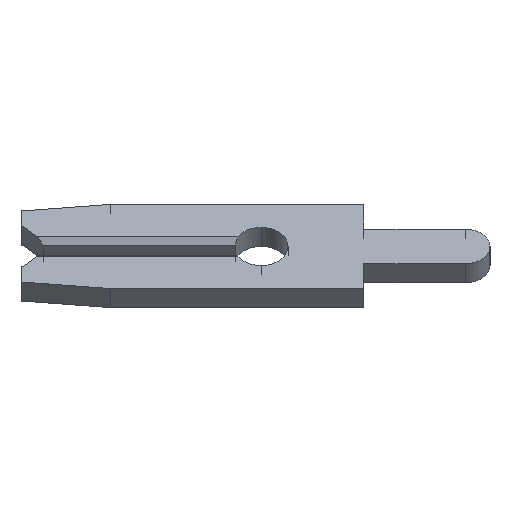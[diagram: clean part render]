
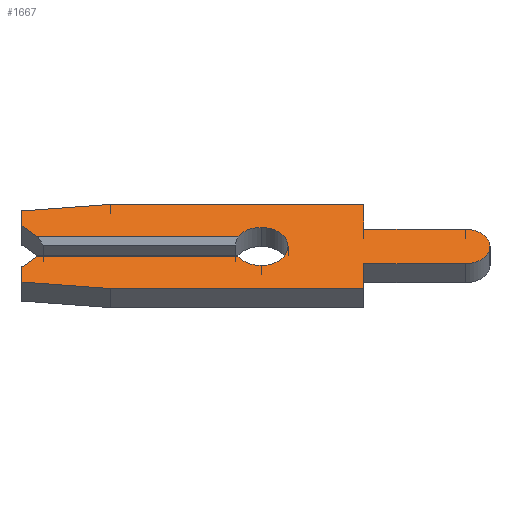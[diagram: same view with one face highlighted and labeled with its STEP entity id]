
A CAD part, left-side view. The second image highlights one B-rep face of the part: STEP entity #1667.
In plain terms, the highlighted face is planar.
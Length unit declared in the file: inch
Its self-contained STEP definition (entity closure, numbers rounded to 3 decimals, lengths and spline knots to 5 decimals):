
#4 = EDGE_CURVE ( 'NONE', #244, #461, #1239, .T. ) ;
#5 = VERTEX_POINT ( 'NONE', #1364 ) ;
#34 = CARTESIAN_POINT ( 'NONE',  ( -0.013, -0.099, -0.0235 ) ) ;
#36 = CARTESIAN_POINT ( 'NONE',  ( -0.013, 0.146, -0.0575 ) ) ;
#54 = VERTEX_POINT ( 'NONE', #1361 ) ;
#83 = EDGE_CURVE ( 'NONE', #1002, #1341, #1536, .T. ) ;
#96 = ORIENTED_EDGE ( 'NONE', *, *, #337, .F. ) ;
#134 = CARTESIAN_POINT ( 'NONE',  ( -0.013, 0.231, 0.028 ) ) ;
#136 = ORIENTED_EDGE ( 'NONE', *, *, #1131, .F. ) ;
#138 = CARTESIAN_POINT ( 'NONE',  ( -0.013, 0.231, 0.04857 ) ) ;
#140 = ORIENTED_EDGE ( 'NONE', *, *, #744, .F. ) ;
#153 = CARTESIAN_POINT ( 'NONE',  ( -0.013, 0., 0. ) ) ;
#181 = EDGE_CURVE ( 'NONE', #1184, #1570, #1102, .T. ) ;
#193 = VERTEX_POINT ( 'NONE', #850 ) ;
#195 = LINE ( 'NONE', #522, #796 ) ;
#197 = DIRECTION ( 'NONE',  ( 0., 0., -1. ) ) ;
#204 = CARTESIAN_POINT ( 'NONE',  ( -0.013, -0.1975, -0.0235 ) ) ;
#235 = ORIENTED_EDGE ( 'NONE', *, *, #1245, .F. ) ;
#244 = VERTEX_POINT ( 'NONE', #204 ) ;
#266 = CARTESIAN_POINT ( 'NONE',  ( -0.013, 0., 0. ) ) ;
#281 = EDGE_CURVE ( 'NONE', #320, #244, #333, .T. ) ;
#283 = ORIENTED_EDGE ( 'NONE', *, *, #181, .F. ) ;
#285 = ORIENTED_EDGE ( 'NONE', *, *, #4, .F. ) ;
#316 = VECTOR ( 'NONE', #1560, 39.37008 ) ;
#320 = VERTEX_POINT ( 'NONE', #1524 ) ;
#322 = LINE ( 'NONE', #1227, #638 ) ;
#330 = EDGE_CURVE ( 'NONE', #461, #592, #766, .T. ) ;
#333 = CIRCLE ( 'NONE', #1401, 0.0235 ) ;
#337 = EDGE_CURVE ( 'NONE', #659, #320, #1081, .T. ) ;
#347 = DIRECTION ( 'NONE',  ( 1., 0., 0. ) ) ;
#358 = LINE ( 'NONE', #507, #316 ) ;
#382 = VECTOR ( 'NONE', #597, 39.37008 ) ;
#411 = VECTOR ( 'NONE', #786, 39.37008 ) ;
#420 = VERTEX_POINT ( 'NONE', #1701 ) ;
#424 = EDGE_CURVE ( 'NONE', #1570, #1647, #358, .T. ) ;
#461 = VERTEX_POINT ( 'NONE', #1427 ) ;
#467 = CARTESIAN_POINT ( 'NONE',  ( -0.013, 0.231, -0.04857 ) ) ;
#479 = DIRECTION ( 'NONE',  ( 1., 0., 0. ) ) ;
#488 = ORIENTED_EDGE ( 'NONE', *, *, #330, .F. ) ;
#490 = LINE ( 'NONE', #134, #1108 ) ;
#505 = CARTESIAN_POINT ( 'NONE',  ( -0.013, 0.216, -0.013 ) ) ;
#507 = CARTESIAN_POINT ( 'NONE',  ( -0.013, 0.231, -0.028 ) ) ;
#515 = LINE ( 'NONE', #138, #574 ) ;
#522 = CARTESIAN_POINT ( 'NONE',  ( -0.013, 0.146, 0.0575 ) ) ;
#531 = DIRECTION ( 'NONE',  ( -1., 0., 0. ) ) ;
#536 = DIRECTION ( 'NONE',  ( 0., 0., -1. ) ) ;
#545 = AXIS2_PLACEMENT_3D ( 'NONE', #936, #1602, #536 ) ;
#570 = CARTESIAN_POINT ( 'NONE',  ( -0.013, 0.231, 0.013 ) ) ;
#574 = VECTOR ( 'NONE', #1463, 39.37008 ) ;
#585 = ORIENTED_EDGE ( 'NONE', *, *, #839, .F. ) ;
#591 = ORIENTED_EDGE ( 'NONE', *, *, #1204, .F. ) ;
#592 = VERTEX_POINT ( 'NONE', #619 ) ;
#597 = DIRECTION ( 'NONE',  ( 0., 0.995, 0.105 ) ) ;
#602 = CARTESIAN_POINT ( 'NONE',  ( -0.013, -0.099, 0.0235 ) ) ;
#619 = CARTESIAN_POINT ( 'NONE',  ( -0.013, -0.099, -0.0575 ) ) ;
#622 = ORIENTED_EDGE ( 'NONE', *, *, #424, .F. ) ;
#638 = VECTOR ( 'NONE', #967, 39.37008 ) ;
#659 = VERTEX_POINT ( 'NONE', #1454 ) ;
#671 = EDGE_CURVE ( 'NONE', #1002, #193, #1617, .T. ) ;
#677 = DIRECTION ( 'NONE',  ( 0., 0., -1. ) ) ;
#680 = ORIENTED_EDGE ( 'NONE', *, *, #1024, .F. ) ;
#689 = CARTESIAN_POINT ( 'NONE',  ( -0.013, 0., -0.026 ) ) ;
#701 = DIRECTION ( 'NONE',  ( 0., -1., 0. ) ) ;
#708 = ORIENTED_EDGE ( 'NONE', *, *, #1312, .F. ) ;
#711 = CIRCLE ( 'NONE', #1095, 0.026 ) ;
#744 = EDGE_CURVE ( 'NONE', #420, #5, #195, .T. ) ;
#766 = LINE ( 'NONE', #1660, #1497 ) ;
#786 = DIRECTION ( 'NONE',  ( 0., 0.707, 0.707 ) ) ;
#794 = CARTESIAN_POINT ( 'NONE',  ( -0.013, 0.231, 0.04857 ) ) ;
#796 = VECTOR ( 'NONE', #823, 39.37008 ) ;
#801 = DIRECTION ( 'NONE',  ( 0., -1., 0. ) ) ;
#819 = DIRECTION ( 'NONE',  ( -1., 0., 0. ) ) ;
#823 = DIRECTION ( 'NONE',  ( 0., -1., 0. ) ) ;
#837 = FACE_OUTER_BOUND ( 'NONE', #1158, .T. ) ;
#839 = EDGE_CURVE ( 'NONE', #5, #659, #902, .T. ) ;
#850 = CARTESIAN_POINT ( 'NONE',  ( -0.013, 0.231, 0.028 ) ) ;
#854 = ORIENTED_EDGE ( 'NONE', *, *, #892, .F. ) ;
#858 = DIRECTION ( 'NONE',  ( 0., 0., -1. ) ) ;
#867 = CARTESIAN_POINT ( 'NONE',  ( -0.013, -0.1975, 0. ) ) ;
#874 = DIRECTION ( 'NONE',  ( 0., -1., 0. ) ) ;
#888 = VECTOR ( 'NONE', #1644, 39.37008 ) ;
#892 = EDGE_CURVE ( 'NONE', #1647, #897, #1071, .T. ) ;
#897 = VERTEX_POINT ( 'NONE', #505 ) ;
#902 = LINE ( 'NONE', #915, #1422 ) ;
#915 = CARTESIAN_POINT ( 'NONE',  ( -0.013, -0.099, 0.0575 ) ) ;
#924 = CARTESIAN_POINT ( 'NONE',  ( -0.013, 0., -0.013 ) ) ;
#936 = CARTESIAN_POINT ( 'NONE',  ( -0.013, 0., 0. ) ) ;
#967 = DIRECTION ( 'NONE',  ( 0., 1., 0. ) ) ;
#1002 = VERTEX_POINT ( 'NONE', #1183 ) ;
#1003 = AXIS2_PLACEMENT_3D ( 'NONE', #266, #531, #677 ) ;
#1021 = ORIENTED_EDGE ( 'NONE', *, *, #1489, .F. ) ;
#1024 = EDGE_CURVE ( 'NONE', #54, #1293, #1650, .T. ) ;
#1048 = VERTEX_POINT ( 'NONE', #1468 ) ;
#1071 = LINE ( 'NONE', #1439, #1272 ) ;
#1076 = EDGE_CURVE ( 'NONE', #1293, #1048, #1505, .T. ) ;
#1081 = LINE ( 'NONE', #602, #1156 ) ;
#1095 = AXIS2_PLACEMENT_3D ( 'NONE', #153, #819, #1636 ) ;
#1102 = LINE ( 'NONE', #1517, #382 ) ;
#1108 = VECTOR ( 'NONE', #1202, 39.37008 ) ;
#1131 = EDGE_CURVE ( 'NONE', #1250, #420, #515, .T. ) ;
#1156 = VECTOR ( 'NONE', #874, 39.37008 ) ;
#1158 = EDGE_LOOP ( 'NONE', ( #1502, #708, #1481, #680, #591, #854, #622, #283, #1021, #488, #285, #1504, #96, #585, #140, #136, #235, #1611 ) ) ;
#1171 = DIRECTION ( 'NONE',  ( 0., 0., -1. ) ) ;
#1183 = CARTESIAN_POINT ( 'NONE',  ( -0.013, 0.216, 0.013 ) ) ;
#1184 = VERTEX_POINT ( 'NONE', #36 ) ;
#1185 = CARTESIAN_POINT ( 'NONE',  ( -0.013, 0.2105, 0.0075 ) ) ;
#1202 = DIRECTION ( 'NONE',  ( 0., 0., 1. ) ) ;
#1204 = EDGE_CURVE ( 'NONE', #897, #54, #1300, .T. ) ;
#1206 = VECTOR ( 'NONE', #701, 39.37008 ) ;
#1227 = CARTESIAN_POINT ( 'NONE',  ( -0.013, 0.146, -0.0575 ) ) ;
#1239 = LINE ( 'NONE', #34, #888 ) ;
#1242 = AXIS2_PLACEMENT_3D ( 'NONE', #1528, #347, #197 ) ;
#1245 = EDGE_CURVE ( 'NONE', #193, #1250, #490, .T. ) ;
#1250 = VERTEX_POINT ( 'NONE', #794 ) ;
#1272 = VECTOR ( 'NONE', #1296, 39.37008 ) ;
#1293 = VERTEX_POINT ( 'NONE', #689 ) ;
#1296 = DIRECTION ( 'NONE',  ( 0., -0.707, 0.707 ) ) ;
#1300 = LINE ( 'NONE', #924, #1594 ) ;
#1312 = EDGE_CURVE ( 'NONE', #1048, #1341, #711, .T. ) ;
#1341 = VERTEX_POINT ( 'NONE', #1623 ) ;
#1361 = CARTESIAN_POINT ( 'NONE',  ( -0.013, 0.02252, -0.013 ) ) ;
#1364 = CARTESIAN_POINT ( 'NONE',  ( -0.013, -0.099, 0.0575 ) ) ;
#1389 = CARTESIAN_POINT ( 'NONE',  ( -0.013, 0.231, -0.028 ) ) ;
#1401 = AXIS2_PLACEMENT_3D ( 'NONE', #867, #479, #1658 ) ;
#1422 = VECTOR ( 'NONE', #1171, 39.37008 ) ;
#1427 = CARTESIAN_POINT ( 'NONE',  ( -0.013, -0.099, -0.0235 ) ) ;
#1439 = CARTESIAN_POINT ( 'NONE',  ( -0.013, 0.2105, -0.0075 ) ) ;
#1454 = CARTESIAN_POINT ( 'NONE',  ( -0.013, -0.099, 0.0235 ) ) ;
#1463 = DIRECTION ( 'NONE',  ( 0., -0.995, 0.105 ) ) ;
#1468 = CARTESIAN_POINT ( 'NONE',  ( -0.013, 0., 0.026 ) ) ;
#1481 = ORIENTED_EDGE ( 'NONE', *, *, #1076, .F. ) ;
#1489 = EDGE_CURVE ( 'NONE', #592, #1184, #322, .T. ) ;
#1497 = VECTOR ( 'NONE', #858, 39.37008 ) ;
#1502 = ORIENTED_EDGE ( 'NONE', *, *, #83, .T. ) ;
#1504 = ORIENTED_EDGE ( 'NONE', *, *, #281, .F. ) ;
#1505 = CIRCLE ( 'NONE', #545, 0.026 ) ;
#1509 = PLANE ( 'NONE',  #1242 ) ;
#1517 = CARTESIAN_POINT ( 'NONE',  ( -0.013, 0.231, -0.04857 ) ) ;
#1524 = CARTESIAN_POINT ( 'NONE',  ( -0.013, -0.1975, 0.0235 ) ) ;
#1528 = CARTESIAN_POINT ( 'NONE',  ( -0.013, 0., 0. ) ) ;
#1536 = LINE ( 'NONE', #570, #1206 ) ;
#1560 = DIRECTION ( 'NONE',  ( 0., 0., 1. ) ) ;
#1570 = VERTEX_POINT ( 'NONE', #467 ) ;
#1594 = VECTOR ( 'NONE', #801, 39.37008 ) ;
#1602 = DIRECTION ( 'NONE',  ( -1., 0., 0. ) ) ;
#1611 = ORIENTED_EDGE ( 'NONE', *, *, #671, .F. ) ;
#1617 = LINE ( 'NONE', #1185, #411 ) ;
#1623 = CARTESIAN_POINT ( 'NONE',  ( -0.013, 0.02252, 0.013 ) ) ;
#1636 = DIRECTION ( 'NONE',  ( 0., 0., -1. ) ) ;
#1644 = DIRECTION ( 'NONE',  ( 0., 1., 0. ) ) ;
#1647 = VERTEX_POINT ( 'NONE', #1389 ) ;
#1650 = CIRCLE ( 'NONE', #1003, 0.026 ) ;
#1658 = DIRECTION ( 'NONE',  ( 0., 0., 1. ) ) ;
#1660 = CARTESIAN_POINT ( 'NONE',  ( -0.013, -0.099, -0.0575 ) ) ;
#1667 = ADVANCED_FACE ( 'NONE', ( #837 ), #1509, .F. ) ;
#1701 = CARTESIAN_POINT ( 'NONE',  ( -0.013, 0.146, 0.0575 ) ) ;
